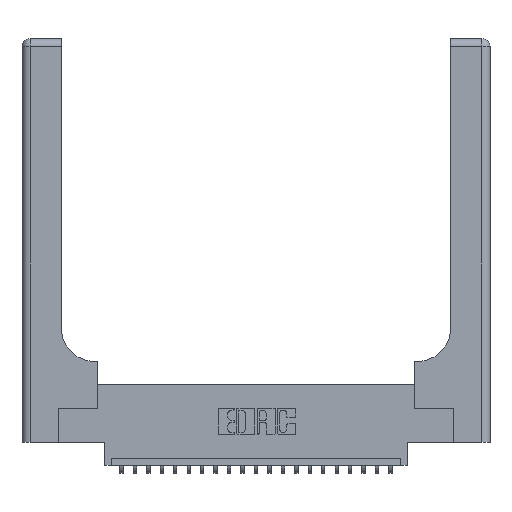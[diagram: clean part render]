
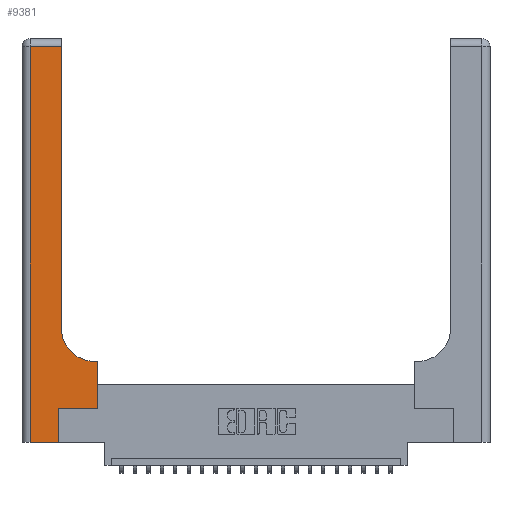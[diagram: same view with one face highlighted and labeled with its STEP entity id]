
A CAD part, top view. The second image highlights one B-rep face of the part: STEP entity #9381.
In plain terms, the highlighted planar face has unit normal (0, 0, 1).
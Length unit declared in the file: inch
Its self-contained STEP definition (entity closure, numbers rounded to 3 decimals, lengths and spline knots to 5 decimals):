
#177 = DIRECTION ( 'NONE',  ( 0., 1., 0. ) ) ;
#245 = LINE ( 'NONE', #4597, #21768 ) ;
#997 = VERTEX_POINT ( 'NONE', #18202 ) ;
#1150 = LINE ( 'NONE', #18691, #7537 ) ;
#1407 = DIRECTION ( 'NONE',  ( 1., 0., 0. ) ) ;
#1461 = EDGE_CURVE ( 'NONE', #10006, #12035, #9227, .T. ) ;
#1490 = LINE ( 'NONE', #16723, #10797 ) ;
#1859 = VERTEX_POINT ( 'NONE', #11214 ) ;
#2389 = ORIENTED_EDGE ( 'NONE', *, *, #7826, .T. ) ;
#2538 = FACE_OUTER_BOUND ( 'NONE', #19975, .T. ) ;
#2557 = VERTEX_POINT ( 'NONE', #10868 ) ;
#3168 = ORIENTED_EDGE ( 'NONE', *, *, #1461, .T. ) ;
#3624 = DIRECTION ( 'NONE',  ( 0., 1., 0. ) ) ;
#4074 = CARTESIAN_POINT ( 'NONE',  ( 0.269, 0.25, 0.37 ) ) ;
#4140 = EDGE_CURVE ( 'NONE', #1859, #23151, #4503, .T. ) ;
#4503 = LINE ( 'NONE', #9939, #15481 ) ;
#4597 = CARTESIAN_POINT ( 'NONE',  ( 0.06, 3., 0.37 ) ) ;
#4647 = ORIENTED_EDGE ( 'NONE', *, *, #16395, .T. ) ;
#5022 = CARTESIAN_POINT ( 'NONE',  ( 0., 3., 0.37 ) ) ;
#5603 = AXIS2_PLACEMENT_3D ( 'NONE', #5022, #21606, #12424 ) ;
#6647 = VECTOR ( 'NONE', #177, 39.37008 ) ;
#6896 = CARTESIAN_POINT ( 'NONE',  ( 0.269, 0., 0.37 ) ) ;
#7327 = CIRCLE ( 'NONE', #10733, 0.25 ) ;
#7537 = VECTOR ( 'NONE', #18787, 39.37008 ) ;
#7643 = VECTOR ( 'NONE', #9272, 39.37008 ) ;
#7826 = EDGE_CURVE ( 'NONE', #9968, #2557, #20611, .T. ) ;
#7935 = VECTOR ( 'NONE', #10271, 39.37008 ) ;
#8323 = ORIENTED_EDGE ( 'NONE', *, *, #19660, .T. ) ;
#8962 = CARTESIAN_POINT ( 'NONE',  ( 0.269, 0., 0.37 ) ) ;
#9227 = LINE ( 'NONE', #8962, #6647 ) ;
#9272 = DIRECTION ( 'NONE',  ( 1., 0., 0. ) ) ;
#9323 = ORIENTED_EDGE ( 'NONE', *, *, #20938, .T. ) ;
#9381 = ADVANCED_FACE ( 'NONE', ( #2538 ), #18101, .F. ) ;
#9939 = CARTESIAN_POINT ( 'NONE',  ( 0., 2.94, 0.37 ) ) ;
#9968 = VERTEX_POINT ( 'NONE', #12442 ) ;
#10006 = VERTEX_POINT ( 'NONE', #6896 ) ;
#10271 = DIRECTION ( 'NONE',  ( 1., 0., 0. ) ) ;
#10733 = AXIS2_PLACEMENT_3D ( 'NONE', #16984, #15934, #1407 ) ;
#10797 = VECTOR ( 'NONE', #3624, 39.37008 ) ;
#10868 = CARTESIAN_POINT ( 'NONE',  ( 0.5415, 0.6, 0.37 ) ) ;
#11214 = CARTESIAN_POINT ( 'NONE',  ( 0.2915, 2.94, 0.37 ) ) ;
#12035 = VERTEX_POINT ( 'NONE', #17825 ) ;
#12424 = DIRECTION ( 'NONE',  ( -1., 0., 0. ) ) ;
#12442 = CARTESIAN_POINT ( 'NONE',  ( 0.5585, 0.6, 0.37 ) ) ;
#12482 = ORIENTED_EDGE ( 'NONE', *, *, #15496, .T. ) ;
#12582 = VERTEX_POINT ( 'NONE', #17506 ) ;
#13474 = CARTESIAN_POINT ( 'NONE',  ( 0.5585, 0.25, 0.37 ) ) ;
#14310 = VERTEX_POINT ( 'NONE', #13474 ) ;
#15106 = CARTESIAN_POINT ( 'NONE',  ( 0.2915, 0.6, 0.37 ) ) ;
#15481 = VECTOR ( 'NONE', #20881, 39.37008 ) ;
#15496 = EDGE_CURVE ( 'NONE', #12035, #14310, #15740, .T. ) ;
#15578 = DIRECTION ( 'NONE',  ( 0., -1., 0. ) ) ;
#15740 = LINE ( 'NONE', #4074, #7643 ) ;
#15934 = DIRECTION ( 'NONE',  ( 0., 0., -1. ) ) ;
#16321 = LINE ( 'NONE', #17777, #7935 ) ;
#16395 = EDGE_CURVE ( 'NONE', #2557, #12582, #7327, .T. ) ;
#16723 = CARTESIAN_POINT ( 'NONE',  ( 0.2915, 3., 0.37 ) ) ;
#16984 = CARTESIAN_POINT ( 'NONE',  ( 0.5415, 0.85, 0.37 ) ) ;
#17506 = CARTESIAN_POINT ( 'NONE',  ( 0.2915, 0.85, 0.37 ) ) ;
#17777 = CARTESIAN_POINT ( 'NONE',  ( 0., 0., 0.37 ) ) ;
#17825 = CARTESIAN_POINT ( 'NONE',  ( 0.269, 0.25, 0.37 ) ) ;
#18101 = PLANE ( 'NONE',  #5603 ) ;
#18202 = CARTESIAN_POINT ( 'NONE',  ( 0.06, 0., 0.37 ) ) ;
#18305 = ORIENTED_EDGE ( 'NONE', *, *, #21329, .T. ) ;
#18691 = CARTESIAN_POINT ( 'NONE',  ( 0.5585, 0.25, 0.37 ) ) ;
#18787 = DIRECTION ( 'NONE',  ( 0., 1., 0. ) ) ;
#19660 = EDGE_CURVE ( 'NONE', #997, #10006, #16321, .T. ) ;
#19975 = EDGE_LOOP ( 'NONE', ( #21391, #22759, #9323, #8323, #3168, #12482, #18305, #2389, #4647 ) ) ;
#20042 = EDGE_CURVE ( 'NONE', #12582, #1859, #1490, .T. ) ;
#20463 = CARTESIAN_POINT ( 'NONE',  ( 0.06, 2.94, 0.37 ) ) ;
#20611 = LINE ( 'NONE', #15106, #22642 ) ;
#20881 = DIRECTION ( 'NONE',  ( -1., 0., 0. ) ) ;
#20938 = EDGE_CURVE ( 'NONE', #23151, #997, #245, .T. ) ;
#21329 = EDGE_CURVE ( 'NONE', #14310, #9968, #1150, .T. ) ;
#21391 = ORIENTED_EDGE ( 'NONE', *, *, #20042, .T. ) ;
#21606 = DIRECTION ( 'NONE',  ( 0., 0., -1. ) ) ;
#21768 = VECTOR ( 'NONE', #15578, 39.37008 ) ;
#22333 = DIRECTION ( 'NONE',  ( -1., 0., 0. ) ) ;
#22642 = VECTOR ( 'NONE', #22333, 39.37008 ) ;
#22759 = ORIENTED_EDGE ( 'NONE', *, *, #4140, .T. ) ;
#23151 = VERTEX_POINT ( 'NONE', #20463 ) ;
